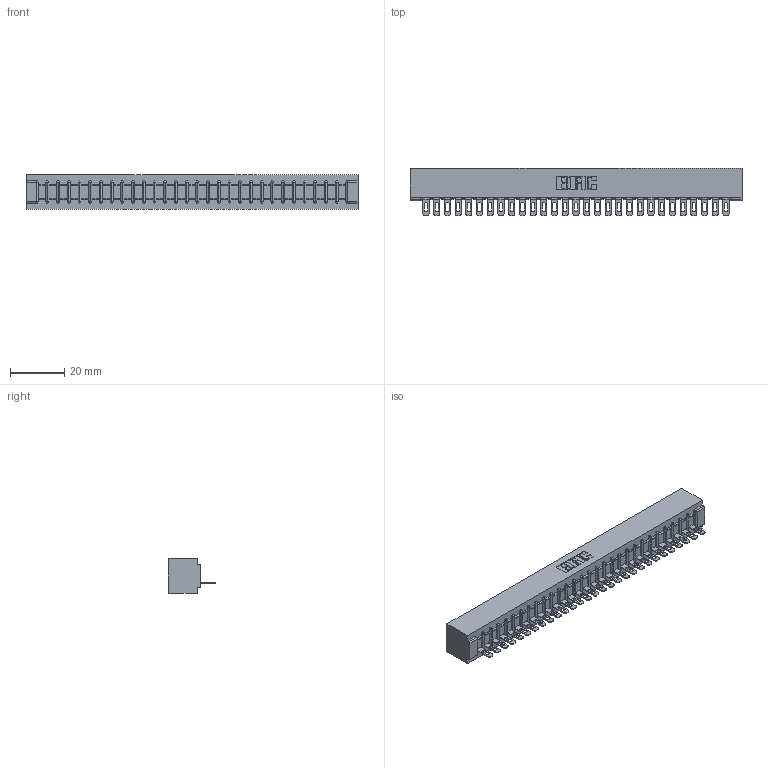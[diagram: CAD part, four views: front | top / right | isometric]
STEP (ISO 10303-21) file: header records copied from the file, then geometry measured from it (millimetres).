
FILE_DESCRIPTION (( 'STEP AP203' ), '1' );
FILE_NAME ('357-029-501-101.STEP', '2018-08-09T07:54:37', ( '' ), ( '' ), 'SwSTEP 2.0', 'SolidWorks 2016', '' );
FILE_SCHEMA (( 'CONFIG_CONTROL_DESIGN' ));
Length unit declared in the file: inch
Products named in the file (3): 307 Part_No Mounting Lugs; 307-290-002_501; 357-029-501-101
Assembly tree (30 placements, depth 2):
  357-029-501-101
    307 Part_No Mounting Lugs
    307-290-002_501  x29
Bounding box: 122.78 x 17.42 x 12.7 mm (x, y, z)
Volume: 13625.5 mm3; surface area: 17393.1 mm2
Topology: 30 solids, 30 shells, 2344 faces, 7201 edges, 4718 vertices
Faces by surface type: plane 1342, cylinder 942, sphere 60
Entity records: 26980 total; most frequent: CARTESIAN_POINT 4548, ORIENTED_EDGE 4538, DIRECTION 4427, EDGE_CURVE 2269, VECTOR 1729, LINE 1729, VERTEX_POINT 1470, AXIS2_PLACEMENT_3D 1349
